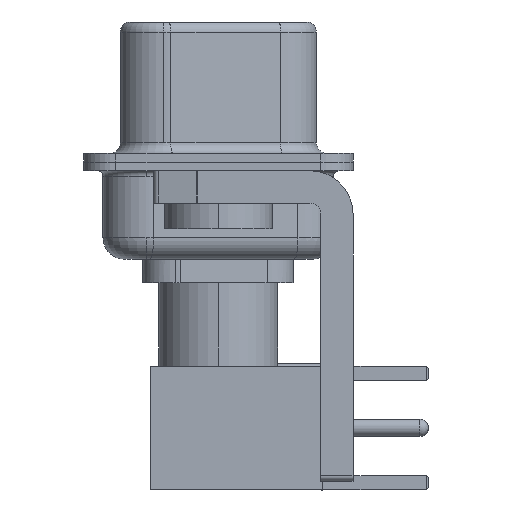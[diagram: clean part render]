
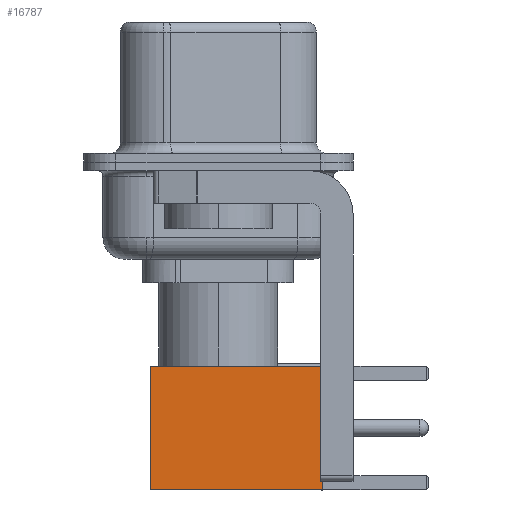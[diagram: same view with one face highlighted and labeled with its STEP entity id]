
A CAD part, left-side view. The second image highlights one B-rep face of the part: STEP entity #16787.
In plain terms, the highlighted face is planar.
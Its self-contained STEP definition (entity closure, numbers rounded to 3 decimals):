
#1314 = CARTESIAN_POINT ( 'NONE',  ( -2.875, 2.875, 8. ) ) ;
#1435 = EDGE_CURVE ( 'NONE', #14326, #16900, #22662, .T. ) ;
#1990 = VECTOR ( 'NONE', #30581, 1000. ) ;
#2374 = ORIENTED_EDGE ( 'NONE', *, *, #1435, .F. ) ;
#2762 = PLANE ( 'NONE',  #25474 ) ;
#3642 = ORIENTED_EDGE ( 'NONE', *, *, #11907, .T. ) ;
#4305 = EDGE_CURVE ( 'NONE', #13101, #14326, #30015, .T. ) ;
#7221 = VECTOR ( 'NONE', #19906, 1000. ) ;
#9387 = LINE ( 'NONE', #20137, #1990 ) ;
#9683 = CARTESIAN_POINT ( 'NONE',  ( -2.875, 2.875, 0. ) ) ;
#11858 = ORIENTED_EDGE ( 'NONE', *, *, #25942, .T. ) ;
#11907 = EDGE_CURVE ( 'NONE', #31989, #16900, #9387, .T. ) ;
#13101 = VERTEX_POINT ( 'NONE', #21124 ) ;
#13195 = CARTESIAN_POINT ( 'NONE',  ( 2.875, 2.875, 0. ) ) ;
#14326 = VERTEX_POINT ( 'NONE', #1314 ) ;
#14333 = DIRECTION ( 'NONE',  ( 0., 0., -1. ) ) ;
#16787 = ADVANCED_FACE ( 'NONE', ( #26188 ), #2762, .T. ) ;
#16900 = VERTEX_POINT ( 'NONE', #24765 ) ;
#17023 = DIRECTION ( 'NONE',  ( -1., 0., 0. ) ) ;
#17514 = LINE ( 'NONE', #25043, #7221 ) ;
#19906 = DIRECTION ( 'NONE',  ( 0., 0., -1. ) ) ;
#20137 = CARTESIAN_POINT ( 'NONE',  ( 0., 2.875, 0. ) ) ;
#21124 = CARTESIAN_POINT ( 'NONE',  ( 2.875, 2.875, 8. ) ) ;
#21605 = VECTOR ( 'NONE', #14333, 1000. ) ;
#22662 = LINE ( 'NONE', #9683, #21605 ) ;
#22796 = CARTESIAN_POINT ( 'NONE',  ( 2.875, 2.875, 0. ) ) ;
#24765 = CARTESIAN_POINT ( 'NONE',  ( -2.875, 2.875, 0. ) ) ;
#25043 = CARTESIAN_POINT ( 'NONE',  ( 2.875, 2.875, 0. ) ) ;
#25474 = AXIS2_PLACEMENT_3D ( 'NONE', #13195, #30796, #25677 ) ;
#25677 = DIRECTION ( 'NONE',  ( 0., 0., 1. ) ) ;
#25942 = EDGE_CURVE ( 'NONE', #13101, #31989, #17514, .T. ) ;
#26188 = FACE_OUTER_BOUND ( 'NONE', #30491, .T. ) ;
#27296 = VECTOR ( 'NONE', #17023, 1000. ) ;
#28117 = CARTESIAN_POINT ( 'NONE',  ( 0., 2.875, 8. ) ) ;
#28152 = ORIENTED_EDGE ( 'NONE', *, *, #4305, .F. ) ;
#30015 = LINE ( 'NONE', #28117, #27296 ) ;
#30491 = EDGE_LOOP ( 'NONE', ( #11858, #3642, #2374, #28152 ) ) ;
#30581 = DIRECTION ( 'NONE',  ( -1., 0., 0. ) ) ;
#30796 = DIRECTION ( 'NONE',  ( 0., 1., 0. ) ) ;
#31989 = VERTEX_POINT ( 'NONE', #22796 ) ;
